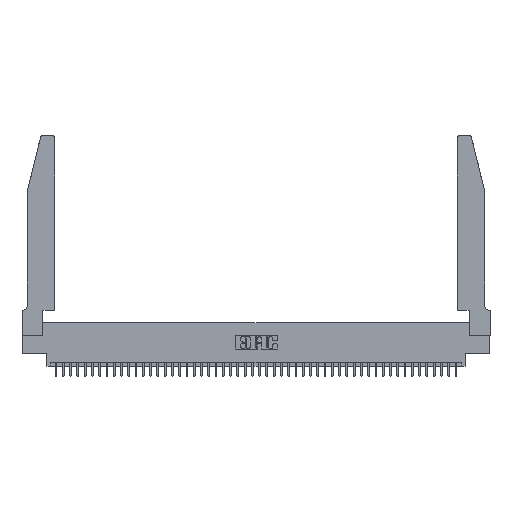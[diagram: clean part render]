
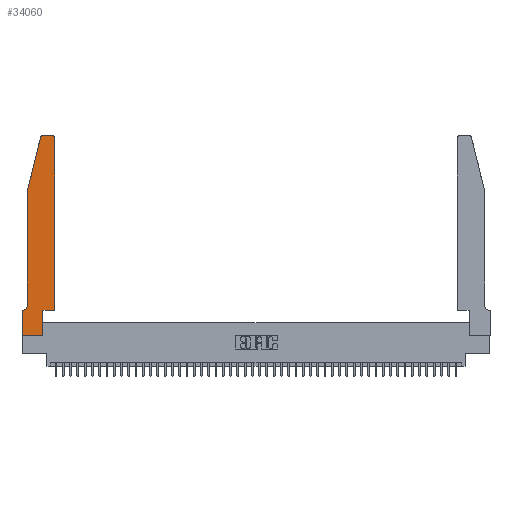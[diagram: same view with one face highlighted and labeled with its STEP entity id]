
A CAD part, top view. The second image highlights one B-rep face of the part: STEP entity #34060.
In plain terms, the highlighted planar face has unit normal (0, 0, 1).
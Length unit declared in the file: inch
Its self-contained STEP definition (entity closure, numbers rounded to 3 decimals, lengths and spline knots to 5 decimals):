
#62 = PLANE ( 'NONE',  #8698 ) ;
#412 = LINE ( 'NONE', #45717, #1012 ) ;
#488 = CIRCLE ( 'NONE', #38664, 0.07 ) ;
#509 = CARTESIAN_POINT ( 'NONE',  ( 0.284, 2.72, 0.37 ) ) ;
#613 = VERTEX_POINT ( 'NONE', #26179 ) ;
#707 = ORIENTED_EDGE ( 'NONE', *, *, #23274, .T. ) ;
#764 = ORIENTED_EDGE ( 'NONE', *, *, #2317, .T. ) ;
#947 = DIRECTION ( 'NONE',  ( -1., 0., 0. ) ) ;
#1012 = VECTOR ( 'NONE', #45138, 39.37008 ) ;
#1050 = DIRECTION ( 'NONE',  ( 1., 0., 0. ) ) ;
#2225 = ORIENTED_EDGE ( 'NONE', *, *, #40037, .T. ) ;
#2317 = EDGE_CURVE ( 'NONE', #14547, #5262, #412, .T. ) ;
#3276 = LINE ( 'NONE', #16384, #23154 ) ;
#3984 = VECTOR ( 'NONE', #5731, 39.37008 ) ;
#4613 = ORIENTED_EDGE ( 'NONE', *, *, #32038, .T. ) ;
#5262 = VERTEX_POINT ( 'NONE', #19961 ) ;
#5473 = DIRECTION ( 'NONE',  ( 0., -1., 0. ) ) ;
#5609 = ORIENTED_EDGE ( 'NONE', *, *, #40624, .T. ) ;
#5631 = CIRCLE ( 'NONE', #29951, 0.03 ) ;
#5731 = DIRECTION ( 'NONE',  ( 1., 0., 0. ) ) ;
#7116 = FACE_OUTER_BOUND ( 'NONE', #23792, .T. ) ;
#7274 = EDGE_CURVE ( 'NONE', #28519, #14547, #26689, .T. ) ;
#7462 = CARTESIAN_POINT ( 'NONE',  ( 0., 0.35, 0.37 ) ) ;
#8141 = CARTESIAN_POINT ( 'NONE',  ( 0.4205, 2.72, 0.37 ) ) ;
#8698 = AXIS2_PLACEMENT_3D ( 'NONE', #7462, #39886, #25384 ) ;
#10140 = VERTEX_POINT ( 'NONE', #19066 ) ;
#10684 = CARTESIAN_POINT ( 'NONE',  ( 0.0755, 2., 0.37 ) ) ;
#10881 = CARTESIAN_POINT ( 'NONE',  ( 0.0055, 0.35, 0.37 ) ) ;
#11984 = CARTESIAN_POINT ( 'NONE',  ( 0., 0., 0.37 ) ) ;
#12447 = ORIENTED_EDGE ( 'NONE', *, *, #17563, .T. ) ;
#13991 = CARTESIAN_POINT ( 'NONE',  ( 0.2865, 0.35, 0.37 ) ) ;
#14547 = VERTEX_POINT ( 'NONE', #39439 ) ;
#14620 = DIRECTION ( 'NONE',  ( 0., -1., 0. ) ) ;
#15400 = EDGE_CURVE ( 'NONE', #30023, #10140, #3276, .T. ) ;
#15708 = CARTESIAN_POINT ( 'NONE',  ( 0.0055, 0.42, 0.37 ) ) ;
#15734 = CARTESIAN_POINT ( 'NONE',  ( 0.0755, 0.42, 0.37 ) ) ;
#15812 = LINE ( 'NONE', #26210, #43105 ) ;
#15937 = VERTEX_POINT ( 'NONE', #15734 ) ;
#16323 = VECTOR ( 'NONE', #14620, 39.37008 ) ;
#16384 = CARTESIAN_POINT ( 'NONE',  ( 0.0755, 0.35, 0.37 ) ) ;
#17563 = EDGE_CURVE ( 'NONE', #613, #23629, #37713, .T. ) ;
#17718 = DIRECTION ( 'NONE',  ( -0.239, -0.971, 0. ) ) ;
#18310 = CARTESIAN_POINT ( 'NONE',  ( 0.2865, 0., 0.37 ) ) ;
#18538 = LINE ( 'NONE', #26479, #32182 ) ;
#18896 = DIRECTION ( 'NONE',  ( 0., 0., -1. ) ) ;
#19066 = CARTESIAN_POINT ( 'NONE',  ( 0., 0.35, 0.37 ) ) ;
#19385 = CARTESIAN_POINT ( 'NONE',  ( 0.4205, 2.75, 0.37 ) ) ;
#19554 = DIRECTION ( 'NONE',  ( -1., 0., 0. ) ) ;
#19572 = ORIENTED_EDGE ( 'NONE', *, *, #23270, .T. ) ;
#19961 = CARTESIAN_POINT ( 'NONE',  ( 0.4505, 2.72, 0.37 ) ) ;
#22573 = DIRECTION ( 'NONE',  ( 1., 0., 0. ) ) ;
#23154 = VECTOR ( 'NONE', #45605, 39.37008 ) ;
#23270 = EDGE_CURVE ( 'NONE', #23986, #613, #5631, .T. ) ;
#23274 = EDGE_CURVE ( 'NONE', #10140, #43790, #15812, .T. ) ;
#23629 = VERTEX_POINT ( 'NONE', #35573 ) ;
#23792 = EDGE_LOOP ( 'NONE', ( #2225, #19572, #12447, #24127, #5609, #25336, #707, #36882, #4613, #33928, #764, #36699 ) ) ;
#23965 = EDGE_CURVE ( 'NONE', #43790, #44277, #28256, .T. ) ;
#23986 = VERTEX_POINT ( 'NONE', #44856 ) ;
#24127 = ORIENTED_EDGE ( 'NONE', *, *, #39861, .T. ) ;
#25336 = ORIENTED_EDGE ( 'NONE', *, *, #15400, .T. ) ;
#25384 = DIRECTION ( 'NONE',  ( 1., 0., 0. ) ) ;
#26179 = CARTESIAN_POINT ( 'NONE',  ( 0.25487, 2.72718, 0.37 ) ) ;
#26210 = CARTESIAN_POINT ( 'NONE',  ( 0., 0., 0.37 ) ) ;
#26479 = CARTESIAN_POINT ( 'NONE',  ( 0.2605, 2.75, 0.37 ) ) ;
#26689 = LINE ( 'NONE', #30968, #3984 ) ;
#28256 = LINE ( 'NONE', #33437, #43003 ) ;
#28519 = VERTEX_POINT ( 'NONE', #45956 ) ;
#28620 = VECTOR ( 'NONE', #17718, 39.37008 ) ;
#29561 = DIRECTION ( 'NONE',  ( 0., 0., 1. ) ) ;
#29951 = AXIS2_PLACEMENT_3D ( 'NONE', #509, #29561, #22573 ) ;
#30023 = VERTEX_POINT ( 'NONE', #10881 ) ;
#30158 = EDGE_CURVE ( 'NONE', #5262, #40099, #33723, .T. ) ;
#30968 = CARTESIAN_POINT ( 'NONE',  ( 0.4505, 0.35, 0.37 ) ) ;
#32007 = AXIS2_PLACEMENT_3D ( 'NONE', #8141, #44184, #37046 ) ;
#32038 = EDGE_CURVE ( 'NONE', #44277, #28519, #44320, .T. ) ;
#32182 = VECTOR ( 'NONE', #19554, 39.37008 ) ;
#33437 = CARTESIAN_POINT ( 'NONE',  ( 0., 0., 0.37 ) ) ;
#33723 = CIRCLE ( 'NONE', #32007, 0.03 ) ;
#33928 = ORIENTED_EDGE ( 'NONE', *, *, #7274, .T. ) ;
#34060 = ADVANCED_FACE ( 'NONE', ( #7116 ), #62, .T. ) ;
#35573 = CARTESIAN_POINT ( 'NONE',  ( 0.0755, 2., 0.37 ) ) ;
#35641 = LINE ( 'NONE', #10684, #16323 ) ;
#36699 = ORIENTED_EDGE ( 'NONE', *, *, #30158, .T. ) ;
#36882 = ORIENTED_EDGE ( 'NONE', *, *, #23965, .T. ) ;
#36992 = VECTOR ( 'NONE', #46711, 39.37008 ) ;
#37046 = DIRECTION ( 'NONE',  ( 1., 0., 0. ) ) ;
#37713 = LINE ( 'NONE', #42951, #28620 ) ;
#38664 = AXIS2_PLACEMENT_3D ( 'NONE', #15708, #18896, #947 ) ;
#39439 = CARTESIAN_POINT ( 'NONE',  ( 0.4505, 0.35, 0.37 ) ) ;
#39861 = EDGE_CURVE ( 'NONE', #23629, #15937, #35641, .T. ) ;
#39886 = DIRECTION ( 'NONE',  ( 0., 0., 1. ) ) ;
#40037 = EDGE_CURVE ( 'NONE', #40099, #23986, #18538, .T. ) ;
#40099 = VERTEX_POINT ( 'NONE', #19385 ) ;
#40624 = EDGE_CURVE ( 'NONE', #15937, #30023, #488, .T. ) ;
#42951 = CARTESIAN_POINT ( 'NONE',  ( 0.0755, 2., 0.37 ) ) ;
#43003 = VECTOR ( 'NONE', #1050, 39.37008 ) ;
#43105 = VECTOR ( 'NONE', #5473, 39.37008 ) ;
#43790 = VERTEX_POINT ( 'NONE', #11984 ) ;
#44184 = DIRECTION ( 'NONE',  ( 0., 0., 1. ) ) ;
#44277 = VERTEX_POINT ( 'NONE', #18310 ) ;
#44320 = LINE ( 'NONE', #13991, #36992 ) ;
#44856 = CARTESIAN_POINT ( 'NONE',  ( 0.284, 2.75, 0.37 ) ) ;
#45138 = DIRECTION ( 'NONE',  ( 0., 1., 0. ) ) ;
#45605 = DIRECTION ( 'NONE',  ( -1., 0., 0. ) ) ;
#45717 = CARTESIAN_POINT ( 'NONE',  ( 0.4505, 0.35, 0.37 ) ) ;
#45956 = CARTESIAN_POINT ( 'NONE',  ( 0.2865, 0.35, 0.37 ) ) ;
#46711 = DIRECTION ( 'NONE',  ( 0., 1., 0. ) ) ;
